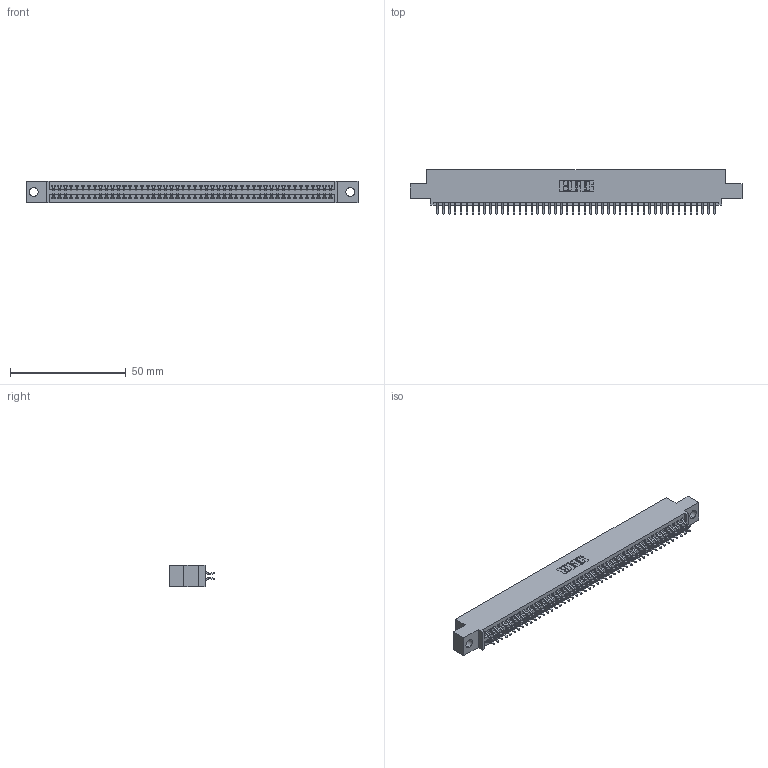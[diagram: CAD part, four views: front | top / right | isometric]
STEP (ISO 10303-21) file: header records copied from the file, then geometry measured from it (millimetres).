
FILE_DESCRIPTION (( 'STEP AP203' ), '1' );
FILE_NAME ('345-096-556-504.STEP', '2021-05-20T17:25:51', ( '' ), ( '' ), 'SwSTEP 2.0', 'SolidWorks 2020', '' );
FILE_SCHEMA (( 'CONFIG_CONTROL_DESIGN' ));
Length unit declared in the file: inch
Products named in the file (3): 345 Part_0.110 Offset - 0.156 Dia-TI; 345-096-556-504; 345-292-001_556 Tail
Assembly tree (97 placements, depth 2):
  345-096-556-504
    345 Part_0.110 Offset - 0.156 Dia-TI
    345-292-001_556 Tail  x96
Bounding box: 143.13 x 19.24 x 9.4 mm (x, y, z)
Volume: 13776.3 mm3; surface area: 20340.2 mm2
Topology: 97 solids, 97 shells, 5520 faces, 16421 edges, 10818 vertices
Faces by surface type: plane 3650, cylinder 1870
Entity records: 37625 total; most frequent: CARTESIAN_POINT 6322, ORIENTED_EDGE 6242, DIRECTION 5553, EDGE_CURVE 3121, VECTOR 2789, LINE 2789, VERTEX_POINT 2078, AXIS2_PLACEMENT_3D 1382
